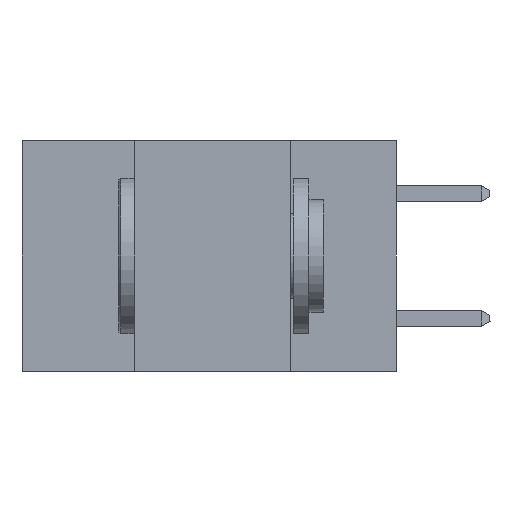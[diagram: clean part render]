
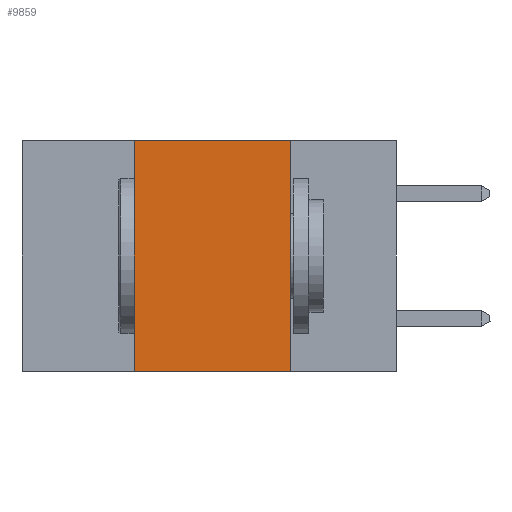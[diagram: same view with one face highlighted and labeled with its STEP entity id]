
A CAD part, left-side view. The second image highlights one B-rep face of the part: STEP entity #9859.
In plain terms, the highlighted planar face has unit normal (-1, 0, 0).
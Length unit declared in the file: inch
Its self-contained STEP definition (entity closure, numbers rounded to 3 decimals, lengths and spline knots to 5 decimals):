
#1331 = LINE ( 'NONE', #22936, #18869 ) ;
#3373 = VERTEX_POINT ( 'NONE', #10963 ) ;
#3840 = LINE ( 'NONE', #4175, #14188 ) ;
#3895 = CARTESIAN_POINT ( 'NONE',  ( 0., 0.17, 0. ) ) ;
#3998 = LINE ( 'NONE', #18675, #15000 ) ;
#4175 = CARTESIAN_POINT ( 'NONE',  ( 0., 0.42, -0.37 ) ) ;
#4544 = CARTESIAN_POINT ( 'NONE',  ( 0., 0.42, 0. ) ) ;
#6293 = PLANE ( 'NONE',  #10754 ) ;
#6980 = EDGE_CURVE ( 'NONE', #14836, #14045, #1331, .T. ) ;
#7023 = VECTOR ( 'NONE', #9113, 39.37008 ) ;
#7667 = DIRECTION ( 'NONE',  ( 0., 0., -1. ) ) ;
#7936 = VERTEX_POINT ( 'NONE', #4544 ) ;
#9113 = DIRECTION ( 'NONE',  ( 0., -1., 0. ) ) ;
#9206 = CARTESIAN_POINT ( 'NONE',  ( 0., 0.6, -0.37 ) ) ;
#9475 = ORIENTED_EDGE ( 'NONE', *, *, #25572, .F. ) ;
#9859 = ADVANCED_FACE ( 'NONE', ( #18573 ), #6293, .F. ) ;
#10723 = DIRECTION ( 'NONE',  ( 0., 0., -1. ) ) ;
#10754 = AXIS2_PLACEMENT_3D ( 'NONE', #28032, #23762, #10723 ) ;
#10963 = CARTESIAN_POINT ( 'NONE',  ( 0., 0.42, -0.37 ) ) ;
#12839 = LINE ( 'NONE', #9206, #7023 ) ;
#14045 = VERTEX_POINT ( 'NONE', #16787 ) ;
#14188 = VECTOR ( 'NONE', #15132, 39.37008 ) ;
#14836 = VERTEX_POINT ( 'NONE', #3895 ) ;
#15000 = VECTOR ( 'NONE', #20893, 39.37008 ) ;
#15132 = DIRECTION ( 'NONE',  ( 0., 0., 1. ) ) ;
#16707 = ORIENTED_EDGE ( 'NONE', *, *, #6980, .F. ) ;
#16787 = CARTESIAN_POINT ( 'NONE',  ( 0., 0.17, -0.37 ) ) ;
#16982 = EDGE_LOOP ( 'NONE', ( #16707, #9475, #23379, #23719 ) ) ;
#18573 = FACE_OUTER_BOUND ( 'NONE', #16982, .T. ) ;
#18675 = CARTESIAN_POINT ( 'NONE',  ( 0., 0.6, 0. ) ) ;
#18869 = VECTOR ( 'NONE', #7667, 39.37008 ) ;
#20893 = DIRECTION ( 'NONE',  ( 0., -1., 0. ) ) ;
#21087 = EDGE_CURVE ( 'NONE', #3373, #14045, #12839, .T. ) ;
#22935 = EDGE_CURVE ( 'NONE', #3373, #7936, #3840, .T. ) ;
#22936 = CARTESIAN_POINT ( 'NONE',  ( 0., 0.17, -0.37 ) ) ;
#23379 = ORIENTED_EDGE ( 'NONE', *, *, #22935, .F. ) ;
#23719 = ORIENTED_EDGE ( 'NONE', *, *, #21087, .T. ) ;
#23762 = DIRECTION ( 'NONE',  ( 1., 0., 0. ) ) ;
#25572 = EDGE_CURVE ( 'NONE', #7936, #14836, #3998, .T. ) ;
#28032 = CARTESIAN_POINT ( 'NONE',  ( 0., 0.6, 0. ) ) ;
